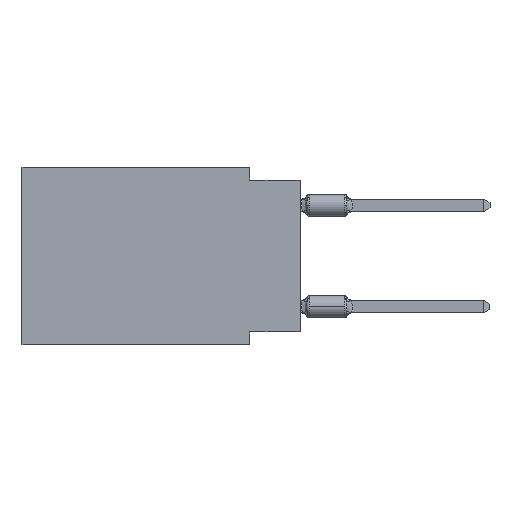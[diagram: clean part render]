
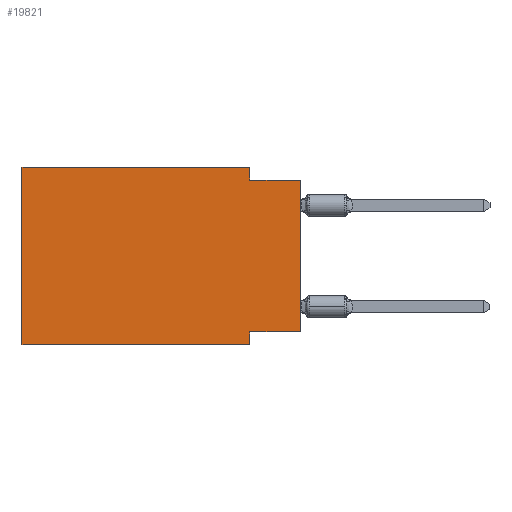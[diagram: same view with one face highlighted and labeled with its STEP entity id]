
A CAD part, left-side view. The second image highlights one B-rep face of the part: STEP entity #19821.
In plain terms, the highlighted planar face has unit normal (-1, 0, 0).
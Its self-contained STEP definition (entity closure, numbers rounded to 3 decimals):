
#66 = EDGE_LOOP ( 'NONE', ( #11424, #7860, #21903, #8189, #16953, #12874, #15066, #9894 ) ) ;
#390 = AXIS2_PLACEMENT_3D ( 'NONE', #13175, #20282, #7826 ) ;
#1083 = DIRECTION ( 'NONE',  ( 0., 0., -1. ) ) ;
#2143 = DIRECTION ( 'NONE',  ( 0., -1., 0. ) ) ;
#2209 = LINE ( 'NONE', #5489, #21026 ) ;
#2430 = FACE_OUTER_BOUND ( 'NONE', #66, .T. ) ;
#2992 = DIRECTION ( 'NONE',  ( 0., -1., 0. ) ) ;
#3054 = EDGE_CURVE ( 'NONE', #3314, #5397, #17619, .T. ) ;
#3176 = CARTESIAN_POINT ( 'NONE',  ( 0., 0., -0.635 ) ) ;
#3287 = LINE ( 'NONE', #14037, #13359 ) ;
#3314 = VERTEX_POINT ( 'NONE', #13300 ) ;
#3588 = EDGE_CURVE ( 'NONE', #10480, #19654, #21429, .T. ) ;
#4121 = CARTESIAN_POINT ( 'NONE',  ( 0., 13.97, 0. ) ) ;
#4924 = EDGE_CURVE ( 'NONE', #19654, #16680, #3287, .T. ) ;
#5397 = VERTEX_POINT ( 'NONE', #17263 ) ;
#5489 = CARTESIAN_POINT ( 'NONE',  ( 0., 13.97, 0. ) ) ;
#5607 = DIRECTION ( 'NONE',  ( 0., 0., 1. ) ) ;
#5657 = CARTESIAN_POINT ( 'NONE',  ( 0., 13.97, -8.89 ) ) ;
#6641 = CARTESIAN_POINT ( 'NONE',  ( 0., 0., -8.255 ) ) ;
#7826 = DIRECTION ( 'NONE',  ( 0., 0., -1. ) ) ;
#7860 = ORIENTED_EDGE ( 'NONE', *, *, #17944, .F. ) ;
#8146 = DIRECTION ( 'NONE',  ( 0., 0., 1. ) ) ;
#8189 = ORIENTED_EDGE ( 'NONE', *, *, #16303, .F. ) ;
#8789 = CARTESIAN_POINT ( 'NONE',  ( 0., 2.54, -8.89 ) ) ;
#9081 = DIRECTION ( 'NONE',  ( 0., 1., 0. ) ) ;
#9894 = ORIENTED_EDGE ( 'NONE', *, *, #3588, .F. ) ;
#10308 = DIRECTION ( 'NONE',  ( 0., -1., 0. ) ) ;
#10480 = VERTEX_POINT ( 'NONE', #6641 ) ;
#11016 = VECTOR ( 'NONE', #8146, 1000. ) ;
#11424 = ORIENTED_EDGE ( 'NONE', *, *, #12192, .T. ) ;
#11543 = PLANE ( 'NONE',  #390 ) ;
#12192 = EDGE_CURVE ( 'NONE', #10480, #19330, #12930, .T. ) ;
#12803 = CARTESIAN_POINT ( 'NONE',  ( 0., 0., -8.255 ) ) ;
#12874 = ORIENTED_EDGE ( 'NONE', *, *, #20035, .T. ) ;
#12930 = LINE ( 'NONE', #20030, #11016 ) ;
#13175 = CARTESIAN_POINT ( 'NONE',  ( 0., 13.97, 0. ) ) ;
#13300 = CARTESIAN_POINT ( 'NONE',  ( 0., 2.54, 0. ) ) ;
#13359 = VECTOR ( 'NONE', #17291, 1000. ) ;
#13479 = VECTOR ( 'NONE', #9081, 1000. ) ;
#14037 = CARTESIAN_POINT ( 'NONE',  ( 0., 2.54, -8.89 ) ) ;
#14455 = EDGE_CURVE ( 'NONE', #15875, #15132, #2209, .T. ) ;
#14507 = CARTESIAN_POINT ( 'NONE',  ( 0., 0., -0.635 ) ) ;
#15066 = ORIENTED_EDGE ( 'NONE', *, *, #4924, .F. ) ;
#15132 = VERTEX_POINT ( 'NONE', #4121 ) ;
#15377 = LINE ( 'NONE', #15609, #16250 ) ;
#15401 = CARTESIAN_POINT ( 'NONE',  ( 0., 13.97, -8.89 ) ) ;
#15609 = CARTESIAN_POINT ( 'NONE',  ( 0., 13.97, 0. ) ) ;
#15875 = VERTEX_POINT ( 'NONE', #15401 ) ;
#16250 = VECTOR ( 'NONE', #2992, 1000. ) ;
#16303 = EDGE_CURVE ( 'NONE', #15132, #3314, #15377, .T. ) ;
#16467 = CARTESIAN_POINT ( 'NONE',  ( 0., 2.54, -8.255 ) ) ;
#16680 = VERTEX_POINT ( 'NONE', #8789 ) ;
#16953 = ORIENTED_EDGE ( 'NONE', *, *, #14455, .F. ) ;
#16967 = CARTESIAN_POINT ( 'NONE',  ( 0., 2.54, 0. ) ) ;
#17263 = CARTESIAN_POINT ( 'NONE',  ( 0., 2.54, -0.635 ) ) ;
#17291 = DIRECTION ( 'NONE',  ( 0., 0., -1. ) ) ;
#17619 = LINE ( 'NONE', #16967, #22652 ) ;
#17944 = EDGE_CURVE ( 'NONE', #5397, #19330, #23011, .T. ) ;
#19330 = VERTEX_POINT ( 'NONE', #14507 ) ;
#19654 = VERTEX_POINT ( 'NONE', #16467 ) ;
#19821 = ADVANCED_FACE ( 'NONE', ( #2430 ), #11543, .F. ) ;
#20030 = CARTESIAN_POINT ( 'NONE',  ( 0., 0., 0. ) ) ;
#20035 = EDGE_CURVE ( 'NONE', #15875, #16680, #21972, .T. ) ;
#20071 = VECTOR ( 'NONE', #10308, 1000. ) ;
#20282 = DIRECTION ( 'NONE',  ( 1., 0., 0. ) ) ;
#21026 = VECTOR ( 'NONE', #5607, 1000. ) ;
#21429 = LINE ( 'NONE', #12803, #13479 ) ;
#21630 = VECTOR ( 'NONE', #2143, 1000. ) ;
#21903 = ORIENTED_EDGE ( 'NONE', *, *, #3054, .F. ) ;
#21972 = LINE ( 'NONE', #5657, #21630 ) ;
#22652 = VECTOR ( 'NONE', #1083, 1000. ) ;
#23011 = LINE ( 'NONE', #3176, #20071 ) ;
